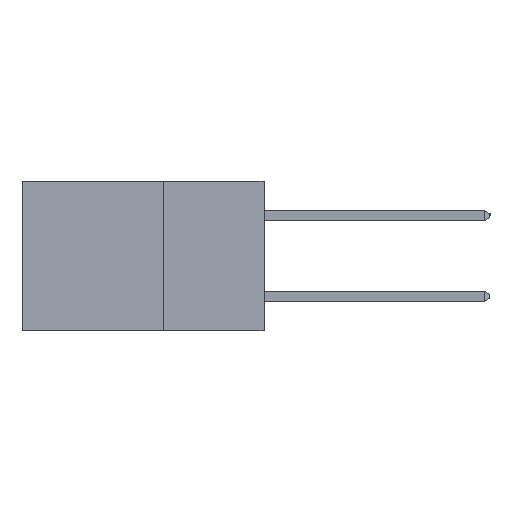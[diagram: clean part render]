
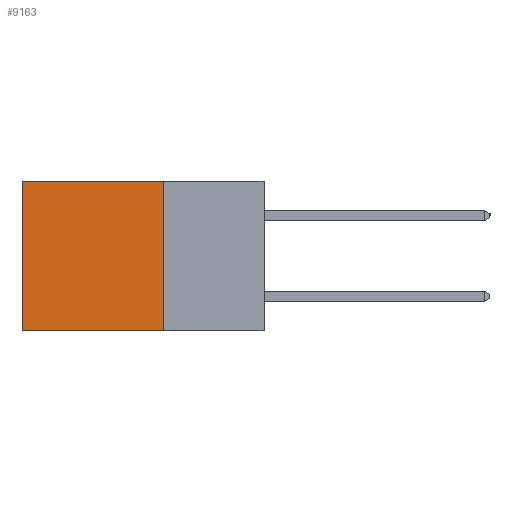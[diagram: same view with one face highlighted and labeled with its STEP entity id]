
A CAD part, left-side view. The second image highlights one B-rep face of the part: STEP entity #9163.
In plain terms, the highlighted planar face has unit normal (-1, 0, 0).
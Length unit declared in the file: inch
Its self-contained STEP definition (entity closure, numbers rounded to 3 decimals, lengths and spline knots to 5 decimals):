
#76 = DIRECTION ( 'NONE',  ( 0., 0., -1. ) ) ;
#80 = LINE ( 'NONE', #937, #2797 ) ;
#937 = CARTESIAN_POINT ( 'NONE',  ( 0.2615, 0.25, -0.37 ) ) ;
#973 = ORIENTED_EDGE ( 'NONE', *, *, #7493, .T. ) ;
#1702 = ORIENTED_EDGE ( 'NONE', *, *, #6649, .F. ) ;
#1805 = VERTEX_POINT ( 'NONE', #1918 ) ;
#1837 = VECTOR ( 'NONE', #6843, 39.37008 ) ;
#1918 = CARTESIAN_POINT ( 'NONE',  ( 0.2615, 0.6, 0. ) ) ;
#1947 = LINE ( 'NONE', #5949, #10805 ) ;
#2797 = VECTOR ( 'NONE', #8826, 39.37008 ) ;
#3250 = CARTESIAN_POINT ( 'NONE',  ( 0.2615, 0.6, -0.37 ) ) ;
#3394 = ORIENTED_EDGE ( 'NONE', *, *, #4212, .T. ) ;
#3553 = VECTOR ( 'NONE', #9618, 39.37008 ) ;
#3909 = AXIS2_PLACEMENT_3D ( 'NONE', #8853, #6846, #11707 ) ;
#4139 = ORIENTED_EDGE ( 'NONE', *, *, #5733, .F. ) ;
#4212 = EDGE_CURVE ( 'NONE', #1805, #5830, #1947, .T. ) ;
#4767 = LINE ( 'NONE', #5823, #3553 ) ;
#4935 = VERTEX_POINT ( 'NONE', #5360 ) ;
#5058 = PLANE ( 'NONE',  #3909 ) ;
#5360 = CARTESIAN_POINT ( 'NONE',  ( 0.2615, 0.25, 0. ) ) ;
#5733 = EDGE_CURVE ( 'NONE', #10813, #5830, #80, .T. ) ;
#5743 = EDGE_LOOP ( 'NONE', ( #3394, #4139, #1702, #973 ) ) ;
#5806 = CARTESIAN_POINT ( 'NONE',  ( 0.2615, 0.25, -0.37 ) ) ;
#5823 = CARTESIAN_POINT ( 'NONE',  ( 0.2615, 0.25, 0. ) ) ;
#5830 = VERTEX_POINT ( 'NONE', #3250 ) ;
#5949 = CARTESIAN_POINT ( 'NONE',  ( 0.2615, 0.6, -0.37 ) ) ;
#6649 = EDGE_CURVE ( 'NONE', #4935, #10813, #11342, .T. ) ;
#6843 = DIRECTION ( 'NONE',  ( 0., 0., -1. ) ) ;
#6846 = DIRECTION ( 'NONE',  ( 1., 0., 0. ) ) ;
#6973 = FACE_OUTER_BOUND ( 'NONE', #5743, .T. ) ;
#7493 = EDGE_CURVE ( 'NONE', #4935, #1805, #4767, .T. ) ;
#8826 = DIRECTION ( 'NONE',  ( 0., 1., 0. ) ) ;
#8853 = CARTESIAN_POINT ( 'NONE',  ( 0.2615, 0.25, -0.37 ) ) ;
#9163 = ADVANCED_FACE ( 'NONE', ( #6973 ), #5058, .F. ) ;
#9618 = DIRECTION ( 'NONE',  ( 0., 1., 0. ) ) ;
#10805 = VECTOR ( 'NONE', #76, 39.37008 ) ;
#10813 = VERTEX_POINT ( 'NONE', #10885 ) ;
#10885 = CARTESIAN_POINT ( 'NONE',  ( 0.2615, 0.25, -0.37 ) ) ;
#11342 = LINE ( 'NONE', #5806, #1837 ) ;
#11707 = DIRECTION ( 'NONE',  ( 0., 0., -1. ) ) ;
